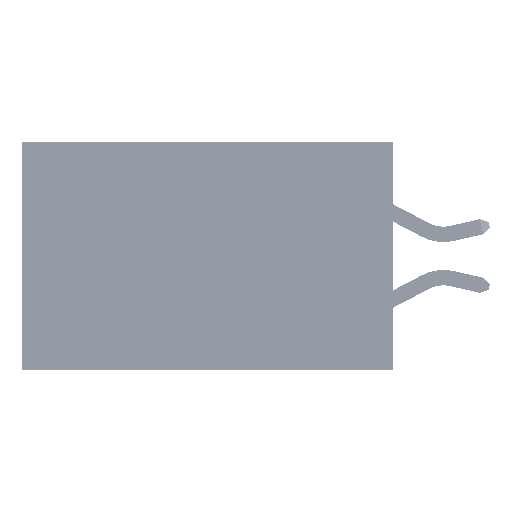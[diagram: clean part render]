
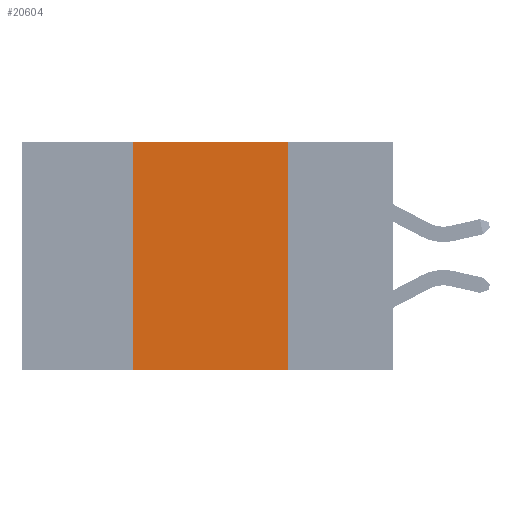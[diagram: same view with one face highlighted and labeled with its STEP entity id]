
A CAD part, left-side view. The second image highlights one B-rep face of the part: STEP entity #20604.
In plain terms, the highlighted planar face has unit normal (-1, 0, 0).
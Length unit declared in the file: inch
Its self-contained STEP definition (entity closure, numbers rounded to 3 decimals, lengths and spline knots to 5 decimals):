
#2849 = AXIS2_PLACEMENT_3D ( 'NONE', #7950, #22788, #4305 ) ;
#4305 = DIRECTION ( 'NONE',  ( 0., 0., -1. ) ) ;
#5151 = VERTEX_POINT ( 'NONE', #6466 ) ;
#6466 = CARTESIAN_POINT ( 'NONE',  ( 0., 0.17, -0.37 ) ) ;
#7597 = VECTOR ( 'NONE', #27035, 39.37008 ) ;
#7950 = CARTESIAN_POINT ( 'NONE',  ( 0., 0.6, 0. ) ) ;
#9330 = VERTEX_POINT ( 'NONE', #12849 ) ;
#9686 = VECTOR ( 'NONE', #19117, 39.37008 ) ;
#12086 = FACE_OUTER_BOUND ( 'NONE', #41119, .T. ) ;
#12430 = CARTESIAN_POINT ( 'NONE',  ( 0., 0.42, 0. ) ) ;
#12849 = CARTESIAN_POINT ( 'NONE',  ( 0., 0.17, 0. ) ) ;
#13864 = LINE ( 'NONE', #45167, #9686 ) ;
#14243 = EDGE_CURVE ( 'NONE', #29572, #5151, #13864, .T. ) ;
#14521 = DIRECTION ( 'NONE',  ( 0., 0., -1. ) ) ;
#16124 = VERTEX_POINT ( 'NONE', #21828 ) ;
#16441 = VECTOR ( 'NONE', #14521, 39.37008 ) ;
#18310 = EDGE_CURVE ( 'NONE', #29572, #16124, #26797, .T. ) ;
#18345 = CARTESIAN_POINT ( 'NONE',  ( 0., 0.6, 0. ) ) ;
#19117 = DIRECTION ( 'NONE',  ( 0., -1., 0. ) ) ;
#20207 = ORIENTED_EDGE ( 'NONE', *, *, #38166, .F. ) ;
#20604 = ADVANCED_FACE ( 'NONE', ( #12086 ), #23264, .F. ) ;
#21828 = CARTESIAN_POINT ( 'NONE',  ( 0., 0.42, 0. ) ) ;
#22788 = DIRECTION ( 'NONE',  ( 1., 0., 0. ) ) ;
#23264 = PLANE ( 'NONE',  #2849 ) ;
#25031 = LINE ( 'NONE', #44479, #16441 ) ;
#26797 = LINE ( 'NONE', #12430, #7597 ) ;
#27035 = DIRECTION ( 'NONE',  ( 0., 0., 1. ) ) ;
#28666 = ORIENTED_EDGE ( 'NONE', *, *, #34669, .F. ) ;
#29572 = VERTEX_POINT ( 'NONE', #45750 ) ;
#34669 = EDGE_CURVE ( 'NONE', #9330, #5151, #25031, .T. ) ;
#36357 = LINE ( 'NONE', #18345, #45318 ) ;
#36672 = ORIENTED_EDGE ( 'NONE', *, *, #18310, .F. ) ;
#38166 = EDGE_CURVE ( 'NONE', #16124, #9330, #36357, .T. ) ;
#41119 = EDGE_LOOP ( 'NONE', ( #28666, #20207, #36672, #47819 ) ) ;
#44479 = CARTESIAN_POINT ( 'NONE',  ( 0., 0.17, 0. ) ) ;
#45167 = CARTESIAN_POINT ( 'NONE',  ( 0., 0.6, -0.37 ) ) ;
#45318 = VECTOR ( 'NONE', #47793, 39.37008 ) ;
#45750 = CARTESIAN_POINT ( 'NONE',  ( 0., 0.42, -0.37 ) ) ;
#47793 = DIRECTION ( 'NONE',  ( 0., -1., 0. ) ) ;
#47819 = ORIENTED_EDGE ( 'NONE', *, *, #14243, .T. ) ;
